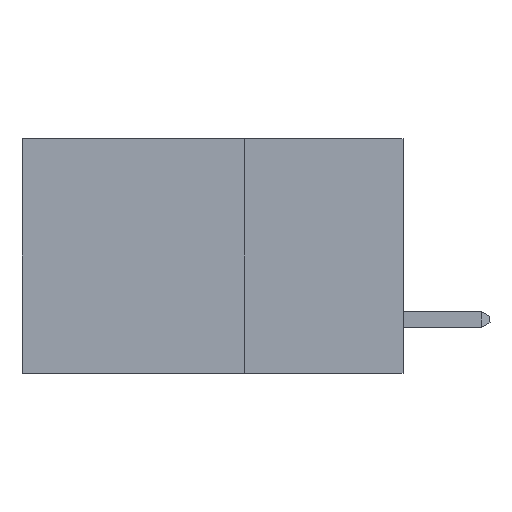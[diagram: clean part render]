
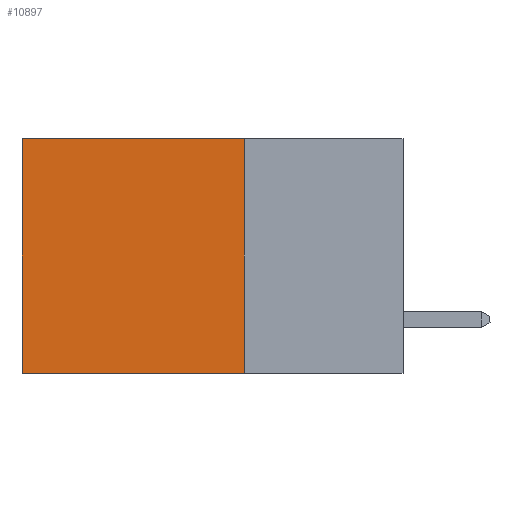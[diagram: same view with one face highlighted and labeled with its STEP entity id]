
A CAD part, left-side view. The second image highlights one B-rep face of the part: STEP entity #10897.
In plain terms, the highlighted planar face has unit normal (-1, 0, 0).
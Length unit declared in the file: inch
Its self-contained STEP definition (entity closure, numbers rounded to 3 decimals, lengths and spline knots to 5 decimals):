
#55 = CARTESIAN_POINT ( 'NONE',  ( 0.2875, 0.6, -0.37 ) ) ;
#170 = DIRECTION ( 'NONE',  ( 0., 0., -1. ) ) ;
#409 = CARTESIAN_POINT ( 'NONE',  ( 0.2875, 0.6, 0. ) ) ;
#859 = DIRECTION ( 'NONE',  ( 0., 1., 0. ) ) ;
#930 = FACE_OUTER_BOUND ( 'NONE', #6653, .T. ) ;
#1800 = ORIENTED_EDGE ( 'NONE', *, *, #4148, .T. ) ;
#1815 = VERTEX_POINT ( 'NONE', #4217 ) ;
#1907 = ORIENTED_EDGE ( 'NONE', *, *, #9033, .F. ) ;
#1986 = ORIENTED_EDGE ( 'NONE', *, *, #5080, .F. ) ;
#2026 = ORIENTED_EDGE ( 'NONE', *, *, #5642, .T. ) ;
#2506 = CARTESIAN_POINT ( 'NONE',  ( 0.2875, 0.25, 0. ) ) ;
#2805 = CARTESIAN_POINT ( 'NONE',  ( 0.2875, 0.25, -0.37 ) ) ;
#2830 = VECTOR ( 'NONE', #7263, 39.37008 ) ;
#2915 = LINE ( 'NONE', #3635, #4765 ) ;
#3455 = DIRECTION ( 'NONE',  ( 0., 0., -1. ) ) ;
#3635 = CARTESIAN_POINT ( 'NONE',  ( 0.2875, 0.25, 0. ) ) ;
#4148 = EDGE_CURVE ( 'NONE', #7256, #7592, #7387, .T. ) ;
#4216 = AXIS2_PLACEMENT_3D ( 'NONE', #4967, #10747, #5855 ) ;
#4217 = CARTESIAN_POINT ( 'NONE',  ( 0.2875, 0.25, 0. ) ) ;
#4765 = VECTOR ( 'NONE', #3455, 39.37008 ) ;
#4967 = CARTESIAN_POINT ( 'NONE',  ( 0.2875, 0.25, 0. ) ) ;
#5080 = EDGE_CURVE ( 'NONE', #1815, #9115, #2915, .T. ) ;
#5642 = EDGE_CURVE ( 'NONE', #1815, #7256, #10335, .T. ) ;
#5855 = DIRECTION ( 'NONE',  ( 0., 0., -1. ) ) ;
#6653 = EDGE_LOOP ( 'NONE', ( #1800, #1907, #1986, #2026 ) ) ;
#6966 = CARTESIAN_POINT ( 'NONE',  ( 0.2875, 0.6, 0. ) ) ;
#7108 = VECTOR ( 'NONE', #170, 39.37008 ) ;
#7256 = VERTEX_POINT ( 'NONE', #6966 ) ;
#7263 = DIRECTION ( 'NONE',  ( 0., 1., 0. ) ) ;
#7387 = LINE ( 'NONE', #409, #7108 ) ;
#7566 = LINE ( 'NONE', #2805, #2830 ) ;
#7592 = VERTEX_POINT ( 'NONE', #55 ) ;
#8013 = VECTOR ( 'NONE', #859, 39.37008 ) ;
#9033 = EDGE_CURVE ( 'NONE', #9115, #7592, #7566, .T. ) ;
#9115 = VERTEX_POINT ( 'NONE', #10526 ) ;
#9974 = PLANE ( 'NONE',  #4216 ) ;
#10335 = LINE ( 'NONE', #2506, #8013 ) ;
#10526 = CARTESIAN_POINT ( 'NONE',  ( 0.2875, 0.25, -0.37 ) ) ;
#10747 = DIRECTION ( 'NONE',  ( 1., 0., 0. ) ) ;
#10897 = ADVANCED_FACE ( 'NONE', ( #930 ), #9974, .F. ) ;
